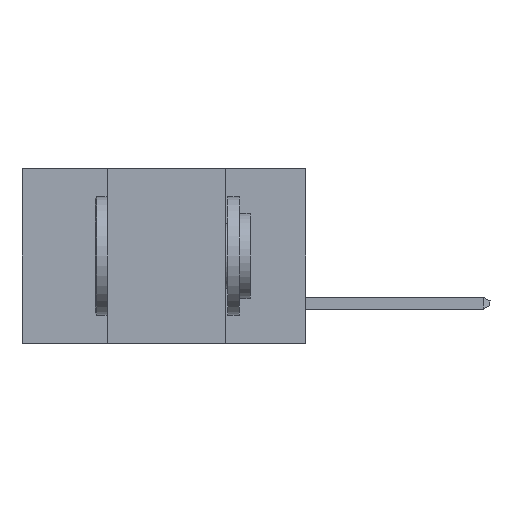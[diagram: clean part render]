
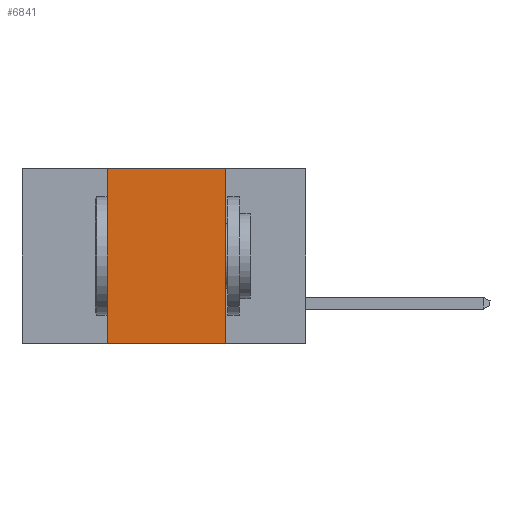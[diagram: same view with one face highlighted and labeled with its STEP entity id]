
A CAD part, left-side view. The second image highlights one B-rep face of the part: STEP entity #6841.
In plain terms, the highlighted planar face has unit normal (-1, 0, 0).
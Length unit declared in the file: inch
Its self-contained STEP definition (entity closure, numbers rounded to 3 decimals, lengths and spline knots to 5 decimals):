
#721 = ORIENTED_EDGE ( 'NONE', *, *, #5968, .F. ) ;
#1465 = CARTESIAN_POINT ( 'NONE',  ( 0., 0.42, -0.37 ) ) ;
#1500 = VECTOR ( 'NONE', #6486, 39.37008 ) ;
#1623 = EDGE_CURVE ( 'NONE', #5075, #6477, #5607, .T. ) ;
#1690 = ORIENTED_EDGE ( 'NONE', *, *, #5020, .F. ) ;
#1709 = DIRECTION ( 'NONE',  ( 1., 0., 0. ) ) ;
#1831 = CARTESIAN_POINT ( 'NONE',  ( 0., 0.42, -0.37 ) ) ;
#2221 = VECTOR ( 'NONE', #8547, 39.37008 ) ;
#2312 = ORIENTED_EDGE ( 'NONE', *, *, #8845, .T. ) ;
#3558 = FACE_OUTER_BOUND ( 'NONE', #7254, .T. ) ;
#3659 = CARTESIAN_POINT ( 'NONE',  ( 0., 0.6, 0. ) ) ;
#3732 = CARTESIAN_POINT ( 'NONE',  ( 0., 0.17, 0. ) ) ;
#3800 = CARTESIAN_POINT ( 'NONE',  ( 0., 0.17, -0.37 ) ) ;
#4845 = ORIENTED_EDGE ( 'NONE', *, *, #1623, .F. ) ;
#5020 = EDGE_CURVE ( 'NONE', #6477, #6562, #10467, .T. ) ;
#5075 = VERTEX_POINT ( 'NONE', #1831 ) ;
#5104 = CARTESIAN_POINT ( 'NONE',  ( 0., 0.6, -0.37 ) ) ;
#5340 = VERTEX_POINT ( 'NONE', #5804 ) ;
#5607 = LINE ( 'NONE', #1465, #8927 ) ;
#5804 = CARTESIAN_POINT ( 'NONE',  ( 0., 0.17, -0.37 ) ) ;
#5833 = LINE ( 'NONE', #5104, #2221 ) ;
#5968 = EDGE_CURVE ( 'NONE', #6562, #5340, #10876, .T. ) ;
#6458 = AXIS2_PLACEMENT_3D ( 'NONE', #3659, #1709, #10407 ) ;
#6477 = VERTEX_POINT ( 'NONE', #8236 ) ;
#6486 = DIRECTION ( 'NONE',  ( 0., 0., -1. ) ) ;
#6551 = DIRECTION ( 'NONE',  ( 0., 0., 1. ) ) ;
#6562 = VERTEX_POINT ( 'NONE', #3732 ) ;
#6841 = ADVANCED_FACE ( 'NONE', ( #3558 ), #6982, .F. ) ;
#6982 = PLANE ( 'NONE',  #6458 ) ;
#7254 = EDGE_LOOP ( 'NONE', ( #721, #1690, #4845, #2312 ) ) ;
#7787 = CARTESIAN_POINT ( 'NONE',  ( 0., 0.6, 0. ) ) ;
#8236 = CARTESIAN_POINT ( 'NONE',  ( 0., 0.42, 0. ) ) ;
#8468 = VECTOR ( 'NONE', #10364, 39.37008 ) ;
#8547 = DIRECTION ( 'NONE',  ( 0., -1., 0. ) ) ;
#8845 = EDGE_CURVE ( 'NONE', #5075, #5340, #5833, .T. ) ;
#8927 = VECTOR ( 'NONE', #6551, 39.37008 ) ;
#10364 = DIRECTION ( 'NONE',  ( 0., -1., 0. ) ) ;
#10407 = DIRECTION ( 'NONE',  ( 0., 0., -1. ) ) ;
#10467 = LINE ( 'NONE', #7787, #8468 ) ;
#10876 = LINE ( 'NONE', #3800, #1500 ) ;
